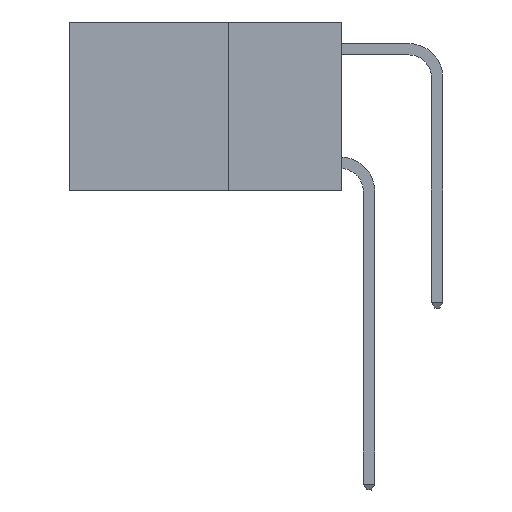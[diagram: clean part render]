
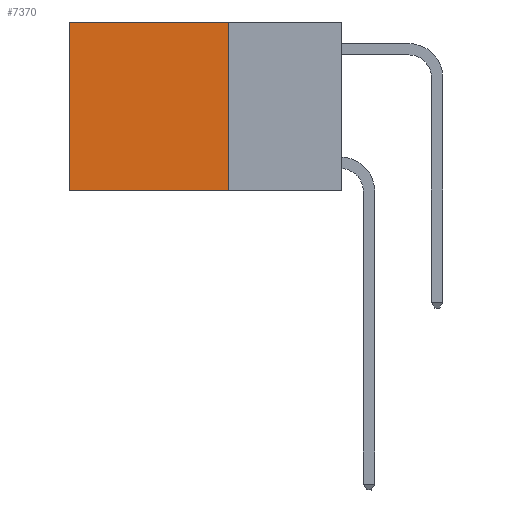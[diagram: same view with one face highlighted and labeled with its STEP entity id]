
A CAD part, left-side view. The second image highlights one B-rep face of the part: STEP entity #7370.
In plain terms, the highlighted planar face has unit normal (-1, 0, 0).
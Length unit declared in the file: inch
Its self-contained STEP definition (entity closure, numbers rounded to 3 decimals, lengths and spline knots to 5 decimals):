
#608 = VERTEX_POINT ( 'NONE', #16755 ) ;
#730 = EDGE_CURVE ( 'NONE', #608, #27824, #828, .T. ) ;
#828 = LINE ( 'NONE', #13938, #5084 ) ;
#2387 = DIRECTION ( 'NONE',  ( 0., 1., 0. ) ) ;
#2629 = DIRECTION ( 'NONE',  ( 0., 0., -1. ) ) ;
#2978 = CARTESIAN_POINT ( 'NONE',  ( 0.2625, 0.6, -0.37 ) ) ;
#3311 = EDGE_CURVE ( 'NONE', #9676, #27824, #13277, .T. ) ;
#4063 = ORIENTED_EDGE ( 'NONE', *, *, #12715, .T. ) ;
#5084 = VECTOR ( 'NONE', #2629, 39.37008 ) ;
#5218 = DIRECTION ( 'NONE',  ( 1., 0., 0. ) ) ;
#7010 = CARTESIAN_POINT ( 'NONE',  ( 0.2625, 0.25, 0. ) ) ;
#7246 = CARTESIAN_POINT ( 'NONE',  ( 0.2625, 0.25, -0.37 ) ) ;
#7370 = ADVANCED_FACE ( 'NONE', ( #9530 ), #18594, .F. ) ;
#7680 = ORIENTED_EDGE ( 'NONE', *, *, #730, .T. ) ;
#9530 = FACE_OUTER_BOUND ( 'NONE', #15998, .T. ) ;
#9676 = VERTEX_POINT ( 'NONE', #7246 ) ;
#10537 = DIRECTION ( 'NONE',  ( 0., 0., -1. ) ) ;
#10890 = DIRECTION ( 'NONE',  ( 0., 1., 0. ) ) ;
#11321 = ORIENTED_EDGE ( 'NONE', *, *, #22023, .F. ) ;
#12715 = EDGE_CURVE ( 'NONE', #26073, #608, #13991, .T. ) ;
#13277 = LINE ( 'NONE', #16484, #24521 ) ;
#13938 = CARTESIAN_POINT ( 'NONE',  ( 0.2625, 0.6, 0. ) ) ;
#13991 = LINE ( 'NONE', #7010, #26781 ) ;
#14145 = DIRECTION ( 'NONE',  ( 0., 0., -1. ) ) ;
#15673 = ORIENTED_EDGE ( 'NONE', *, *, #3311, .F. ) ;
#15998 = EDGE_LOOP ( 'NONE', ( #7680, #15673, #11321, #4063 ) ) ;
#16484 = CARTESIAN_POINT ( 'NONE',  ( 0.2625, 0.25, -0.37 ) ) ;
#16651 = AXIS2_PLACEMENT_3D ( 'NONE', #27684, #5218, #14145 ) ;
#16755 = CARTESIAN_POINT ( 'NONE',  ( 0.2625, 0.6, 0. ) ) ;
#18594 = PLANE ( 'NONE',  #16651 ) ;
#19156 = CARTESIAN_POINT ( 'NONE',  ( 0.2625, 0.25, 0. ) ) ;
#19613 = LINE ( 'NONE', #19156, #22475 ) ;
#22023 = EDGE_CURVE ( 'NONE', #26073, #9676, #19613, .T. ) ;
#22475 = VECTOR ( 'NONE', #10537, 39.37008 ) ;
#24521 = VECTOR ( 'NONE', #10890, 39.37008 ) ;
#26073 = VERTEX_POINT ( 'NONE', #29353 ) ;
#26781 = VECTOR ( 'NONE', #2387, 39.37008 ) ;
#27684 = CARTESIAN_POINT ( 'NONE',  ( 0.2625, 0.25, 0. ) ) ;
#27824 = VERTEX_POINT ( 'NONE', #2978 ) ;
#29353 = CARTESIAN_POINT ( 'NONE',  ( 0.2625, 0.25, 0. ) ) ;
